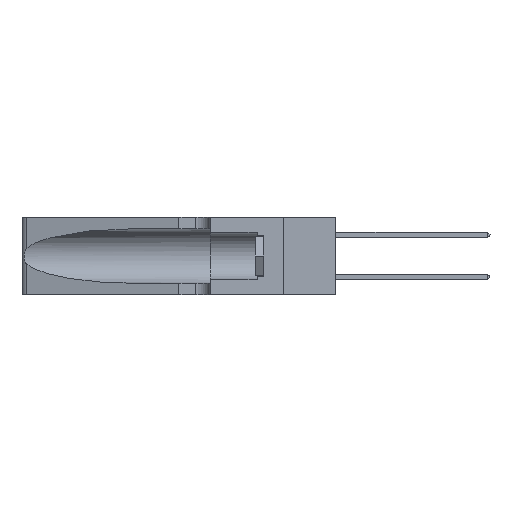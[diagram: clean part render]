
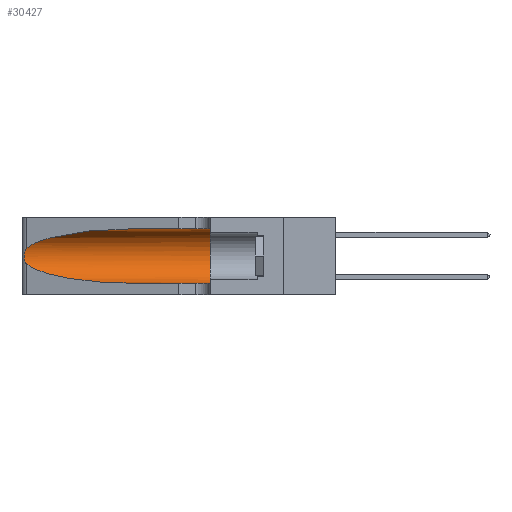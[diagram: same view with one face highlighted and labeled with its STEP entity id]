
A CAD part, left-side view. The second image highlights one B-rep face of the part: STEP entity #30427.
In plain terms, the highlighted cylindrical face has radius 3.308 mm (diameter 6.617 mm), a partial arc.
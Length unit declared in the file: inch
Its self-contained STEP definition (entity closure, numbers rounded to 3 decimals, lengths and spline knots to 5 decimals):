
#561 = VERTEX_POINT ( 'NONE', #21522 ) ;
#885 = CARTESIAN_POINT ( 'NONE',  ( 0.25487, 1.22718, 0.22369 ) ) ;
#1258 = DIRECTION ( 'NONE',  ( 0., 1., 0. ) ) ;
#1278 = CARTESIAN_POINT ( 'NONE',  ( 0.1305, 1.61858, 0.185 ) ) ;
#1899 =( BOUNDED_CURVE ( )  B_SPLINE_CURVE ( 3, ( #13726, #8487, #31631, #18388 ),
 .UNSPECIFIED., .F., .T. ) 
 B_SPLINE_CURVE_WITH_KNOTS ( ( 4, 4 ),
 ( 1.5708, 2.84003 ),
 .UNSPECIFIED. ) 
 CURVE ( )  GEOMETRIC_REPRESENTATION_ITEM ( )  RATIONAL_B_SPLINE_CURVE ( ( 1., 0.87, 0.87, 1. ) ) 
 REPRESENTATION_ITEM ( '' )  );
#2130 = VECTOR ( 'NONE', #8439, 39.37008 ) ;
#2900 = LINE ( 'NONE', #11140, #2130 ) ;
#3258 = CARTESIAN_POINT ( 'NONE',  ( 0.26075, 1.23896, 0.178 ) ) ;
#3629 = VERTEX_POINT ( 'NONE', #18944 ) ;
#3694 = CARTESIAN_POINT ( 'NONE',  ( 0.1305, 0.72297, 0.05475 ) ) ;
#3708 = CARTESIAN_POINT ( 'NONE',  ( 0.25639, 1.23186, 0.15144 ) ) ;
#4474 = ORIENTED_EDGE ( 'NONE', *, *, #31048, .T. ) ;
#4528 = CIRCLE ( 'NONE', #17641, 0.13025 ) ;
#5344 =( BOUNDED_CURVE ( )  B_SPLINE_CURVE ( 3, ( #22787, #25965, #18394, #30787 ),
 .UNSPECIFIED., .F., .T. ) 
 B_SPLINE_CURVE_WITH_KNOTS ( ( 4, 4 ),
 ( 3.44316, 4.71239 ),
 .UNSPECIFIED. ) 
 CURVE ( )  GEOMETRIC_REPRESENTATION_ITEM ( )  RATIONAL_B_SPLINE_CURVE ( ( 1., 0.87, 0.87, 1. ) ) 
 REPRESENTATION_ITEM ( '' )  );
#5824 = VERTEX_POINT ( 'NONE', #28513 ) ;
#8405 = CARTESIAN_POINT ( 'NONE',  ( 0.25555, 1.22994, 0.2215 ) ) ;
#8439 = DIRECTION ( 'NONE',  ( 0., -1., 0. ) ) ;
#8487 = CARTESIAN_POINT ( 'NONE',  ( 0.18966, 0.96281, 0.31525 ) ) ;
#8917 = CARTESIAN_POINT ( 'NONE',  ( 0.1305, 0.35, 0.31525 ) ) ;
#9248 = VERTEX_POINT ( 'NONE', #13065 ) ;
#11069 = CARTESIAN_POINT ( 'NONE',  ( 0.26018, 1.23835, 0.19895 ) ) ;
#11140 = CARTESIAN_POINT ( 'NONE',  ( 0.1305, 1.61858, 0.31525 ) ) ;
#11417 = CARTESIAN_POINT ( 'NONE',  ( 0.25789, 1.23486, 0.15765 ) ) ;
#11456 = DIRECTION ( 'NONE',  ( 0., -1., 0. ) ) ;
#11538 = DIRECTION ( 'NONE',  ( 0., -1., 0. ) ) ;
#12344 = B_SPLINE_CURVE_WITH_KNOTS ( 'NONE', 3,
 ( #885, #8405, #18616, #31788, #28768, #11069, #21550, #3258, #28989, #31549, #11417, #3708, #16305, #29104 ),
 .UNSPECIFIED., .F., .F.,
 ( 4, 2, 2, 2, 2, 2, 4 ),
 ( 0., 0.00027, 0.00053, 0.00107, 0.0016, 0.00187, 0.00214 ),
 .UNSPECIFIED. ) ;
#12445 = VECTOR ( 'NONE', #11538, 39.37008 ) ;
#13065 = CARTESIAN_POINT ( 'NONE',  ( 0.1305, 0.35, 0.05475 ) ) ;
#13638 = CYLINDRICAL_SURFACE ( 'NONE', #24294, 0.13025 ) ;
#13726 = CARTESIAN_POINT ( 'NONE',  ( 0.1305, 0.72297, 0.31525 ) ) ;
#14002 = LINE ( 'NONE', #26778, #12445 ) ;
#16305 = CARTESIAN_POINT ( 'NONE',  ( 0.25555, 1.22993, 0.14849 ) ) ;
#17294 = EDGE_CURVE ( 'NONE', #23050, #9248, #4528, .T. ) ;
#17387 = EDGE_CURVE ( 'NONE', #5824, #23050, #2900, .T. ) ;
#17641 = AXIS2_PLACEMENT_3D ( 'NONE', #24362, #1258, #26453 ) ;
#18388 = CARTESIAN_POINT ( 'NONE',  ( 0.25487, 1.22718, 0.22369 ) ) ;
#18394 = CARTESIAN_POINT ( 'NONE',  ( 0.18966, 0.96281, 0.05475 ) ) ;
#18616 = CARTESIAN_POINT ( 'NONE',  ( 0.25639, 1.23184, 0.21858 ) ) ;
#18944 = CARTESIAN_POINT ( 'NONE',  ( 0.25487, 1.22718, 0.14631 ) ) ;
#19646 = ORIENTED_EDGE ( 'NONE', *, *, #23114, .T. ) ;
#19885 = EDGE_LOOP ( 'NONE', ( #28225, #30413, #19646, #4474, #32095, #30740 ) ) ;
#21151 = EDGE_CURVE ( 'NONE', #561, #3629, #12344, .T. ) ;
#21522 = CARTESIAN_POINT ( 'NONE',  ( 0.25487, 1.22718, 0.22369 ) ) ;
#21550 = CARTESIAN_POINT ( 'NONE',  ( 0.26075, 1.23896, 0.19203 ) ) ;
#22787 = CARTESIAN_POINT ( 'NONE',  ( 0.25487, 1.22718, 0.14631 ) ) ;
#23050 = VERTEX_POINT ( 'NONE', #8917 ) ;
#23114 = EDGE_CURVE ( 'NONE', #3629, #28628, #5344, .T. ) ;
#24294 = AXIS2_PLACEMENT_3D ( 'NONE', #1278, #11456, #31717 ) ;
#24362 = CARTESIAN_POINT ( 'NONE',  ( 0.1305, 0.35, 0.185 ) ) ;
#25965 = CARTESIAN_POINT ( 'NONE',  ( 0.2373, 1.15595, 0.08982 ) ) ;
#26453 = DIRECTION ( 'NONE',  ( 0., 0., 1. ) ) ;
#26778 = CARTESIAN_POINT ( 'NONE',  ( 0.1305, 1.61858, 0.05475 ) ) ;
#28036 = FACE_OUTER_BOUND ( 'NONE', #19885, .T. ) ;
#28225 = ORIENTED_EDGE ( 'NONE', *, *, #31596, .T. ) ;
#28513 = CARTESIAN_POINT ( 'NONE',  ( 0.1305, 0.72297, 0.31525 ) ) ;
#28628 = VERTEX_POINT ( 'NONE', #3694 ) ;
#28768 = CARTESIAN_POINT ( 'NONE',  ( 0.25854, 1.2359, 0.20912 ) ) ;
#28989 = CARTESIAN_POINT ( 'NONE',  ( 0.26017, 1.23833, 0.17102 ) ) ;
#29104 = CARTESIAN_POINT ( 'NONE',  ( 0.25487, 1.22718, 0.14631 ) ) ;
#30413 = ORIENTED_EDGE ( 'NONE', *, *, #21151, .T. ) ;
#30427 = ADVANCED_FACE ( 'NONE', ( #28036 ), #13638, .F. ) ;
#30740 = ORIENTED_EDGE ( 'NONE', *, *, #17387, .F. ) ;
#30787 = CARTESIAN_POINT ( 'NONE',  ( 0.1305, 0.72297, 0.05475 ) ) ;
#31048 = EDGE_CURVE ( 'NONE', #28628, #9248, #14002, .T. ) ;
#31549 = CARTESIAN_POINT ( 'NONE',  ( 0.25856, 1.23593, 0.16098 ) ) ;
#31596 = EDGE_CURVE ( 'NONE', #5824, #561, #1899, .T. ) ;
#31631 = CARTESIAN_POINT ( 'NONE',  ( 0.2373, 1.15595, 0.28018 ) ) ;
#31717 = DIRECTION ( 'NONE',  ( 0., 0., -1. ) ) ;
#31788 = CARTESIAN_POINT ( 'NONE',  ( 0.25787, 1.23484, 0.2124 ) ) ;
#32095 = ORIENTED_EDGE ( 'NONE', *, *, #17294, .F. ) ;
